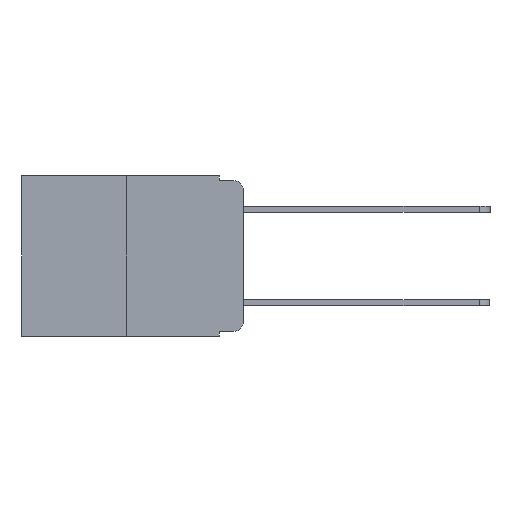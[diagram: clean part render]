
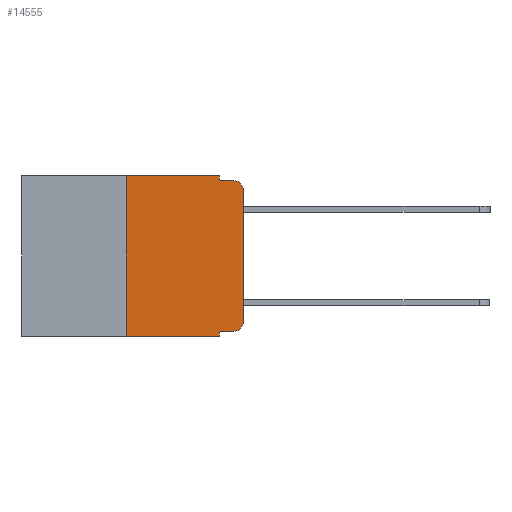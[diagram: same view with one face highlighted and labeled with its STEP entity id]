
A CAD part, left-side view. The second image highlights one B-rep face of the part: STEP entity #14555.
In plain terms, the highlighted planar face has unit normal (-1, 0, 0).
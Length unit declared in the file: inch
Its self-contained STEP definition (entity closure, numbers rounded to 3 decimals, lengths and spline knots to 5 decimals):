
#239 = ORIENTED_EDGE ( 'NONE', *, *, #15143, .T. ) ;
#282 = ORIENTED_EDGE ( 'NONE', *, *, #7654, .T. ) ;
#353 = CARTESIAN_POINT ( 'NONE',  ( 0., 0.051, 0. ) ) ;
#444 = ORIENTED_EDGE ( 'NONE', *, *, #2847, .F. ) ;
#730 = VERTEX_POINT ( 'NONE', #12756 ) ;
#755 = ORIENTED_EDGE ( 'NONE', *, *, #13604, .F. ) ;
#883 = DIRECTION ( 'NONE',  ( 0., -1., 0. ) ) ;
#926 = CARTESIAN_POINT ( 'NONE',  ( 0., 0., 0. ) ) ;
#945 = ORIENTED_EDGE ( 'NONE', *, *, #12156, .F. ) ;
#966 = VECTOR ( 'NONE', #2142, 39.37008 ) ;
#967 = ORIENTED_EDGE ( 'NONE', *, *, #16507, .F. ) ;
#1119 = ORIENTED_EDGE ( 'NONE', *, *, #7623, .T. ) ;
#1418 = VERTEX_POINT ( 'NONE', #9056 ) ;
#1460 = ORIENTED_EDGE ( 'NONE', *, *, #6746, .F. ) ;
#1621 = ORIENTED_EDGE ( 'NONE', *, *, #1943, .T. ) ;
#1755 = ORIENTED_EDGE ( 'NONE', *, *, #20292, .T. ) ;
#1943 = EDGE_CURVE ( 'NONE', #19669, #10925, #3561, .T. ) ;
#1946 = AXIS2_PLACEMENT_3D ( 'NONE', #10348, #22103, #12125 ) ;
#2142 = DIRECTION ( 'NONE',  ( 0., 0., -1. ) ) ;
#2277 = VECTOR ( 'NONE', #9767, 39.37008 ) ;
#2489 = AXIS2_PLACEMENT_3D ( 'NONE', #21754, #16910, #6479 ) ;
#2847 = EDGE_CURVE ( 'NONE', #7336, #10464, #22282, .T. ) ;
#2927 = DIRECTION ( 'NONE',  ( 0., -1., 0. ) ) ;
#3007 = VERTEX_POINT ( 'NONE', #12880 ) ;
#3561 = LINE ( 'NONE', #11062, #16429 ) ;
#3615 = VERTEX_POINT ( 'NONE', #10418 ) ;
#3707 = VECTOR ( 'NONE', #15212, 39.37008 ) ;
#4062 = VECTOR ( 'NONE', #9145, 39.37008 ) ;
#4206 = LINE ( 'NONE', #15443, #8383 ) ;
#6265 = LINE ( 'NONE', #353, #966 ) ;
#6479 = DIRECTION ( 'NONE',  ( 0., 0., -1. ) ) ;
#6746 = EDGE_CURVE ( 'NONE', #19669, #15766, #8429, .T. ) ;
#7208 = CARTESIAN_POINT ( 'NONE',  ( 0., 0.051, 0. ) ) ;
#7265 = CARTESIAN_POINT ( 'NONE',  ( 0., 0.051, -0.333 ) ) ;
#7336 = VERTEX_POINT ( 'NONE', #18044 ) ;
#7532 = DIRECTION ( 'NONE',  ( -1., 0., 0. ) ) ;
#7623 = EDGE_CURVE ( 'NONE', #3615, #15766, #4206, .T. ) ;
#7654 = EDGE_CURVE ( 'NONE', #3007, #10464, #17055, .T. ) ;
#8108 = PLANE ( 'NONE',  #2489 ) ;
#8383 = VECTOR ( 'NONE', #21967, 39.37008 ) ;
#8429 = LINE ( 'NONE', #7208, #3707 ) ;
#8641 = VECTOR ( 'NONE', #17263, 39.37008 ) ;
#9056 = CARTESIAN_POINT ( 'NONE',  ( 0., 0., -0.313 ) ) ;
#9145 = DIRECTION ( 'NONE',  ( 0., -1., 0. ) ) ;
#9252 = EDGE_LOOP ( 'NONE', ( #239, #282, #444, #755, #945, #967, #1119, #1460, #1621, #1755 ) ) ;
#9767 = DIRECTION ( 'NONE',  ( 0., 0., 1. ) ) ;
#10348 = CARTESIAN_POINT ( 'NONE',  ( 0., 0.02, -0.03 ) ) ;
#10418 = CARTESIAN_POINT ( 'NONE',  ( 0., 0.25, -0.343 ) ) ;
#10440 = CARTESIAN_POINT ( 'NONE',  ( 0., 0.25, 0. ) ) ;
#10464 = VERTEX_POINT ( 'NONE', #12145 ) ;
#10925 = VERTEX_POINT ( 'NONE', #21672 ) ;
#11062 = CARTESIAN_POINT ( 'NONE',  ( 0., 0.051, -0.333 ) ) ;
#12125 = DIRECTION ( 'NONE',  ( 0., 0., -1. ) ) ;
#12145 = CARTESIAN_POINT ( 'NONE',  ( 0., 0.02, -0.01 ) ) ;
#12156 = EDGE_CURVE ( 'NONE', #18969, #730, #15327, .T. ) ;
#12605 = AXIS2_PLACEMENT_3D ( 'NONE', #17868, #7532, #19518 ) ;
#12756 = CARTESIAN_POINT ( 'NONE',  ( 0., 0.051, 0. ) ) ;
#12880 = CARTESIAN_POINT ( 'NONE',  ( 0., 0., -0.03 ) ) ;
#13593 = CARTESIAN_POINT ( 'NONE',  ( 0., 0.051, -0.343 ) ) ;
#13604 = EDGE_CURVE ( 'NONE', #730, #7336, #6265, .T. ) ;
#14247 = VECTOR ( 'NONE', #2927, 39.37008 ) ;
#14491 = CARTESIAN_POINT ( 'NONE',  ( 0., 0.051, -0.01 ) ) ;
#14555 = ADVANCED_FACE ( 'NONE', ( #22217 ), #8108, .F. ) ;
#14714 = LINE ( 'NONE', #926, #2277 ) ;
#14925 = CIRCLE ( 'NONE', #12605, 0.02 ) ;
#15143 = EDGE_CURVE ( 'NONE', #1418, #3007, #14714, .T. ) ;
#15212 = DIRECTION ( 'NONE',  ( 0., 0., -1. ) ) ;
#15327 = LINE ( 'NONE', #21770, #14247 ) ;
#15443 = CARTESIAN_POINT ( 'NONE',  ( 0., 0.473, -0.343 ) ) ;
#15766 = VERTEX_POINT ( 'NONE', #13593 ) ;
#16429 = VECTOR ( 'NONE', #883, 39.37008 ) ;
#16507 = EDGE_CURVE ( 'NONE', #3615, #18969, #18323, .T. ) ;
#16910 = DIRECTION ( 'NONE',  ( 1., 0., 0. ) ) ;
#17055 = CIRCLE ( 'NONE', #1946, 0.02 ) ;
#17263 = DIRECTION ( 'NONE',  ( 0., 0., 1. ) ) ;
#17868 = CARTESIAN_POINT ( 'NONE',  ( 0., 0.02, -0.313 ) ) ;
#18044 = CARTESIAN_POINT ( 'NONE',  ( 0., 0.051, -0.01 ) ) ;
#18323 = LINE ( 'NONE', #10440, #8641 ) ;
#18969 = VERTEX_POINT ( 'NONE', #20770 ) ;
#19518 = DIRECTION ( 'NONE',  ( 0., 0., -1. ) ) ;
#19669 = VERTEX_POINT ( 'NONE', #7265 ) ;
#20292 = EDGE_CURVE ( 'NONE', #10925, #1418, #14925, .T. ) ;
#20770 = CARTESIAN_POINT ( 'NONE',  ( 0., 0.25, 0. ) ) ;
#21672 = CARTESIAN_POINT ( 'NONE',  ( 0., 0.02, -0.333 ) ) ;
#21754 = CARTESIAN_POINT ( 'NONE',  ( 0., 0.473, 0. ) ) ;
#21770 = CARTESIAN_POINT ( 'NONE',  ( 0., 0.473, 0. ) ) ;
#21967 = DIRECTION ( 'NONE',  ( 0., -1., 0. ) ) ;
#22103 = DIRECTION ( 'NONE',  ( -1., 0., 0. ) ) ;
#22217 = FACE_OUTER_BOUND ( 'NONE', #9252, .T. ) ;
#22282 = LINE ( 'NONE', #14491, #4062 ) ;
